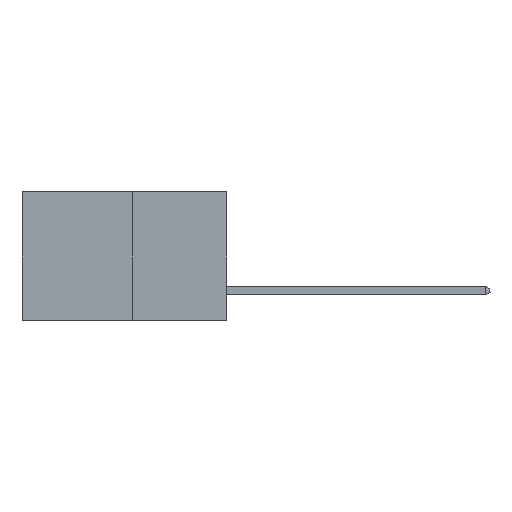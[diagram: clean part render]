
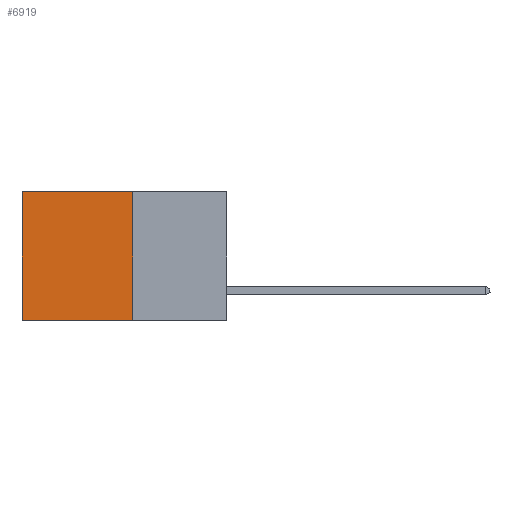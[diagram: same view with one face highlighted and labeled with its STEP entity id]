
A CAD part, left-side view. The second image highlights one B-rep face of the part: STEP entity #6919.
In plain terms, the highlighted planar face has unit normal (-1, 0, 0).
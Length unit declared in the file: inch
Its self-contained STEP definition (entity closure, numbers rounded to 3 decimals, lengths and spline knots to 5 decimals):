
#1258 = LINE ( 'NONE', #9583, #10942 ) ;
#1394 = VERTEX_POINT ( 'NONE', #5065 ) ;
#1531 = VECTOR ( 'NONE', #13106, 39.37008 ) ;
#2161 = CARTESIAN_POINT ( 'NONE',  ( 0.277, 0.27, -0.37 ) ) ;
#2226 = EDGE_CURVE ( 'NONE', #2561, #5976, #2293, .T. ) ;
#2293 = LINE ( 'NONE', #13078, #1531 ) ;
#2561 = VERTEX_POINT ( 'NONE', #6248 ) ;
#3414 = DIRECTION ( 'NONE',  ( 0., 0., -1. ) ) ;
#3759 = VECTOR ( 'NONE', #11986, 39.37008 ) ;
#4329 = AXIS2_PLACEMENT_3D ( 'NONE', #2161, #10663, #3414 ) ;
#4743 = VERTEX_POINT ( 'NONE', #7519 ) ;
#5065 = CARTESIAN_POINT ( 'NONE',  ( 0.277, 0.59, 0. ) ) ;
#5239 = EDGE_CURVE ( 'NONE', #1394, #5976, #12958, .T. ) ;
#5281 = VECTOR ( 'NONE', #7352, 39.37008 ) ;
#5855 = PLANE ( 'NONE',  #4329 ) ;
#5976 = VERTEX_POINT ( 'NONE', #7889 ) ;
#6248 = CARTESIAN_POINT ( 'NONE',  ( 0.277, 0.27, -0.37 ) ) ;
#6919 = ADVANCED_FACE ( 'NONE', ( #13570 ), #5855, .F. ) ;
#7352 = DIRECTION ( 'NONE',  ( 0., 1., 0. ) ) ;
#7519 = CARTESIAN_POINT ( 'NONE',  ( 0.277, 0.27, 0. ) ) ;
#7889 = CARTESIAN_POINT ( 'NONE',  ( 0.277, 0.59, -0.37 ) ) ;
#9583 = CARTESIAN_POINT ( 'NONE',  ( 0.277, 0.27, -0.37 ) ) ;
#9799 = EDGE_LOOP ( 'NONE', ( #14171, #14296, #10814, #14551 ) ) ;
#10094 = EDGE_CURVE ( 'NONE', #4743, #1394, #11656, .T. ) ;
#10663 = DIRECTION ( 'NONE',  ( 1., 0., 0. ) ) ;
#10814 = ORIENTED_EDGE ( 'NONE', *, *, #14903, .F. ) ;
#10832 = CARTESIAN_POINT ( 'NONE',  ( 0.277, 0.59, -0.37 ) ) ;
#10942 = VECTOR ( 'NONE', #15491, 39.37008 ) ;
#11656 = LINE ( 'NONE', #13245, #5281 ) ;
#11986 = DIRECTION ( 'NONE',  ( 0., 0., -1. ) ) ;
#12958 = LINE ( 'NONE', #10832, #3759 ) ;
#13078 = CARTESIAN_POINT ( 'NONE',  ( 0.277, 0.27, -0.37 ) ) ;
#13106 = DIRECTION ( 'NONE',  ( 0., 1., 0. ) ) ;
#13245 = CARTESIAN_POINT ( 'NONE',  ( 0.277, 0.27, 0. ) ) ;
#13570 = FACE_OUTER_BOUND ( 'NONE', #9799, .T. ) ;
#14171 = ORIENTED_EDGE ( 'NONE', *, *, #5239, .T. ) ;
#14296 = ORIENTED_EDGE ( 'NONE', *, *, #2226, .F. ) ;
#14551 = ORIENTED_EDGE ( 'NONE', *, *, #10094, .T. ) ;
#14903 = EDGE_CURVE ( 'NONE', #4743, #2561, #1258, .T. ) ;
#15491 = DIRECTION ( 'NONE',  ( 0., 0., -1. ) ) ;
